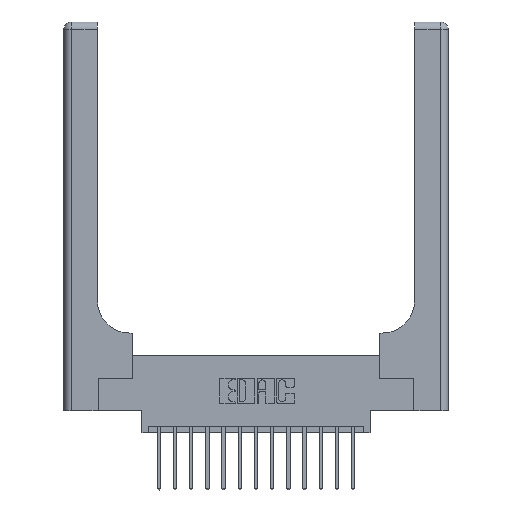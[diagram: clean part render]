
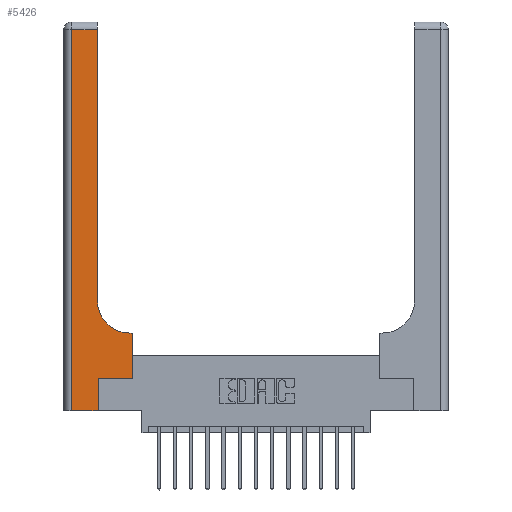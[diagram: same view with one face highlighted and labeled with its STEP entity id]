
A CAD part, top view. The second image highlights one B-rep face of the part: STEP entity #5426.
In plain terms, the highlighted planar face has unit normal (0, 0, 1).
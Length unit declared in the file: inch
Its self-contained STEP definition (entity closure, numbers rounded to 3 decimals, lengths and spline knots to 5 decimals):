
#350 = DIRECTION ( 'NONE',  ( 0., 0., -1. ) ) ;
#433 = EDGE_CURVE ( 'NONE', #1141, #12963, #12437, .T. ) ;
#679 = DIRECTION ( 'NONE',  ( 0., 1., 0. ) ) ;
#919 = LINE ( 'NONE', #3377, #7810 ) ;
#964 = CARTESIAN_POINT ( 'NONE',  ( 0.26, 2.94, 0.37 ) ) ;
#976 = CARTESIAN_POINT ( 'NONE',  ( 0.265, 0., 0.37 ) ) ;
#1139 = VECTOR ( 'NONE', #3594, 39.37008 ) ;
#1141 = VERTEX_POINT ( 'NONE', #9555 ) ;
#1622 = LINE ( 'NONE', #4584, #8557 ) ;
#1833 = DIRECTION ( 'NONE',  ( 1., 0., 0. ) ) ;
#1974 = DIRECTION ( 'NONE',  ( 1., 0., 0. ) ) ;
#2190 = DIRECTION ( 'NONE',  ( 0., 0., -1. ) ) ;
#2369 = CARTESIAN_POINT ( 'NONE',  ( 0.51, 0.85, 0.37 ) ) ;
#2421 = ORIENTED_EDGE ( 'NONE', *, *, #4440, .T. ) ;
#2439 = CARTESIAN_POINT ( 'NONE',  ( 0.26, 0.85, 0.37 ) ) ;
#2681 = VERTEX_POINT ( 'NONE', #976 ) ;
#3113 = LINE ( 'NONE', #10127, #13653 ) ;
#3274 = VECTOR ( 'NONE', #7352, 39.37008 ) ;
#3360 = LINE ( 'NONE', #4835, #17052 ) ;
#3377 = CARTESIAN_POINT ( 'NONE',  ( 0.265, 0., 0.37 ) ) ;
#3594 = DIRECTION ( 'NONE',  ( -1., 0., 0. ) ) ;
#3611 = VECTOR ( 'NONE', #10020, 39.37008 ) ;
#3685 = ORIENTED_EDGE ( 'NONE', *, *, #15272, .T. ) ;
#3834 = VERTEX_POINT ( 'NONE', #10358 ) ;
#3903 = ORIENTED_EDGE ( 'NONE', *, *, #11717, .T. ) ;
#4124 = ORIENTED_EDGE ( 'NONE', *, *, #433, .T. ) ;
#4157 = CARTESIAN_POINT ( 'NONE',  ( 0.528, 0.6, 0.37 ) ) ;
#4440 = EDGE_CURVE ( 'NONE', #10849, #16063, #1622, .T. ) ;
#4487 = AXIS2_PLACEMENT_3D ( 'NONE', #7200, #350, #10014 ) ;
#4584 = CARTESIAN_POINT ( 'NONE',  ( 0.265, 0.25, 0.37 ) ) ;
#4602 = DIRECTION ( 'NONE',  ( 0., 1., 0. ) ) ;
#4835 = CARTESIAN_POINT ( 'NONE',  ( 0.528, 0.25, 0.37 ) ) ;
#5426 = ADVANCED_FACE ( 'NONE', ( #11735 ), #12646, .F. ) ;
#5512 = EDGE_CURVE ( 'NONE', #12963, #8750, #3113, .T. ) ;
#6196 = EDGE_CURVE ( 'NONE', #2681, #10849, #919, .T. ) ;
#7135 = ORIENTED_EDGE ( 'NONE', *, *, #5512, .T. ) ;
#7200 = CARTESIAN_POINT ( 'NONE',  ( 0., 3., 0.37 ) ) ;
#7352 = DIRECTION ( 'NONE',  ( 1., 0., 0. ) ) ;
#7575 = ORIENTED_EDGE ( 'NONE', *, *, #9647, .T. ) ;
#7697 = CARTESIAN_POINT ( 'NONE',  ( 0., 2.94, 0.37 ) ) ;
#7810 = VECTOR ( 'NONE', #679, 39.37008 ) ;
#8043 = LINE ( 'NONE', #7697, #1139 ) ;
#8450 = VERTEX_POINT ( 'NONE', #16601 ) ;
#8557 = VECTOR ( 'NONE', #1833, 39.37008 ) ;
#8750 = VERTEX_POINT ( 'NONE', #964 ) ;
#9555 = CARTESIAN_POINT ( 'NONE',  ( 0.51, 0.6, 0.37 ) ) ;
#9647 = EDGE_CURVE ( 'NONE', #3834, #8450, #17061, .T. ) ;
#9772 = ORIENTED_EDGE ( 'NONE', *, *, #17155, .T. ) ;
#9820 = DIRECTION ( 'NONE',  ( 0., -1., 0. ) ) ;
#9861 = VECTOR ( 'NONE', #9820, 39.37008 ) ;
#9961 = CARTESIAN_POINT ( 'NONE',  ( 0.265, 0.25, 0.37 ) ) ;
#10014 = DIRECTION ( 'NONE',  ( -1., 0., 0. ) ) ;
#10020 = DIRECTION ( 'NONE',  ( -1., 0., 0. ) ) ;
#10127 = CARTESIAN_POINT ( 'NONE',  ( 0.26, 3., 0.37 ) ) ;
#10246 = VERTEX_POINT ( 'NONE', #4157 ) ;
#10358 = CARTESIAN_POINT ( 'NONE',  ( 0.06, 2.94, 0.37 ) ) ;
#10849 = VERTEX_POINT ( 'NONE', #9961 ) ;
#11717 = EDGE_CURVE ( 'NONE', #8750, #3834, #8043, .T. ) ;
#11735 = FACE_OUTER_BOUND ( 'NONE', #12064, .T. ) ;
#12064 = EDGE_LOOP ( 'NONE', ( #7135, #3903, #7575, #12119, #16125, #2421, #9772, #3685, #4124 ) ) ;
#12119 = ORIENTED_EDGE ( 'NONE', *, *, #13347, .T. ) ;
#12437 = CIRCLE ( 'NONE', #17432, 0.25 ) ;
#12517 = CARTESIAN_POINT ( 'NONE',  ( 0.06, 3., 0.37 ) ) ;
#12646 = PLANE ( 'NONE',  #4487 ) ;
#12905 = LINE ( 'NONE', #16774, #3611 ) ;
#12963 = VERTEX_POINT ( 'NONE', #2439 ) ;
#12986 = LINE ( 'NONE', #16901, #3274 ) ;
#13347 = EDGE_CURVE ( 'NONE', #8450, #2681, #12986, .T. ) ;
#13631 = CARTESIAN_POINT ( 'NONE',  ( 0.528, 0.25, 0.37 ) ) ;
#13653 = VECTOR ( 'NONE', #4602, 39.37008 ) ;
#14465 = DIRECTION ( 'NONE',  ( 0., 1., 0. ) ) ;
#15272 = EDGE_CURVE ( 'NONE', #10246, #1141, #12905, .T. ) ;
#16063 = VERTEX_POINT ( 'NONE', #13631 ) ;
#16125 = ORIENTED_EDGE ( 'NONE', *, *, #6196, .T. ) ;
#16601 = CARTESIAN_POINT ( 'NONE',  ( 0.06, 0., 0.37 ) ) ;
#16774 = CARTESIAN_POINT ( 'NONE',  ( 0.26, 0.6, 0.37 ) ) ;
#16901 = CARTESIAN_POINT ( 'NONE',  ( 0., 0., 0.37 ) ) ;
#17052 = VECTOR ( 'NONE', #14465, 39.37008 ) ;
#17061 = LINE ( 'NONE', #12517, #9861 ) ;
#17155 = EDGE_CURVE ( 'NONE', #16063, #10246, #3360, .T. ) ;
#17432 = AXIS2_PLACEMENT_3D ( 'NONE', #2369, #2190, #1974 ) ;
